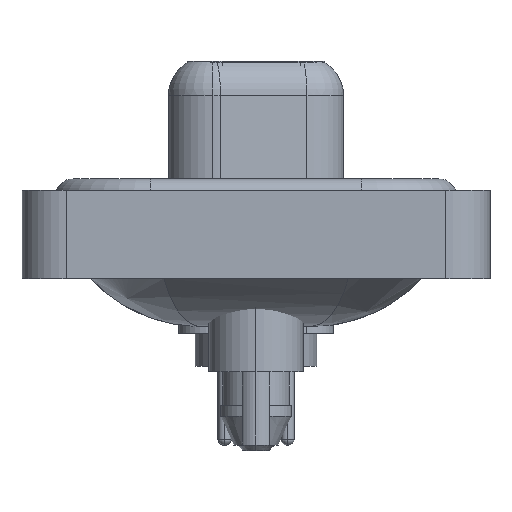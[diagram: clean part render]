
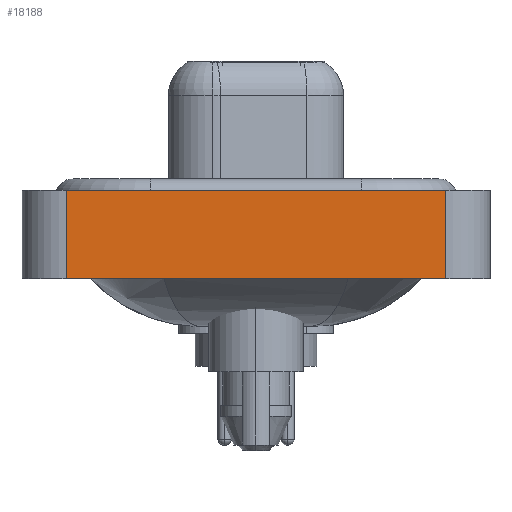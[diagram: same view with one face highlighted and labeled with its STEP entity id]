
A CAD part, left-side view. The second image highlights one B-rep face of the part: STEP entity #18188.
In plain terms, the highlighted planar face has unit normal (-1, 0, 0).
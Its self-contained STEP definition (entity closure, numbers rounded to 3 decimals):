
#572 = LINE ( 'NONE', #20078, #4988 ) ;
#747 = CARTESIAN_POINT ( 'NONE',  ( -7.3, -8.55, -3.6 ) ) ;
#1135 = DIRECTION ( 'NONE',  ( -1., 0., 0. ) ) ;
#1387 = ORIENTED_EDGE ( 'NONE', *, *, #3869, .F. ) ;
#1895 = ORIENTED_EDGE ( 'NONE', *, *, #16898, .T. ) ;
#2384 = CARTESIAN_POINT ( 'NONE',  ( -7.3, -8.55, -3.6 ) ) ;
#3869 = EDGE_CURVE ( 'NONE', #11544, #11591, #7584, .T. ) ;
#3979 = DIRECTION ( 'NONE',  ( 0., -1., 0. ) ) ;
#4447 = DIRECTION ( 'NONE',  ( 0., 0., 1. ) ) ;
#4988 = VECTOR ( 'NONE', #10005, 1000. ) ;
#5085 = DIRECTION ( 'NONE',  ( 0., 0., 1. ) ) ;
#5237 = EDGE_CURVE ( 'NONE', #11591, #5528, #572, .T. ) ;
#5300 = CARTESIAN_POINT ( 'NONE',  ( -7.3, -8.55, -3.6 ) ) ;
#5528 = VERTEX_POINT ( 'NONE', #17703 ) ;
#5994 = VECTOR ( 'NONE', #3979, 1000. ) ;
#6463 = EDGE_CURVE ( 'NONE', #11544, #11216, #18640, .T. ) ;
#7112 = ORIENTED_EDGE ( 'NONE', *, *, #6463, .T. ) ;
#7418 = VECTOR ( 'NONE', #5085, 1000. ) ;
#7584 = LINE ( 'NONE', #10889, #20304 ) ;
#7925 = ORIENTED_EDGE ( 'NONE', *, *, #5237, .F. ) ;
#8734 = LINE ( 'NONE', #5300, #7418 ) ;
#8889 = CARTESIAN_POINT ( 'NONE',  ( -7.3, 8.55, 0.4 ) ) ;
#10005 = DIRECTION ( 'NONE',  ( 0., -1., 0. ) ) ;
#10889 = CARTESIAN_POINT ( 'NONE',  ( -7.3, 8.55, -3.6 ) ) ;
#11216 = VERTEX_POINT ( 'NONE', #2384 ) ;
#11544 = VERTEX_POINT ( 'NONE', #13918 ) ;
#11591 = VERTEX_POINT ( 'NONE', #8889 ) ;
#13786 = FACE_OUTER_BOUND ( 'NONE', #17816, .T. ) ;
#13918 = CARTESIAN_POINT ( 'NONE',  ( -7.3, 8.55, -3.6 ) ) ;
#14002 = DIRECTION ( 'NONE',  ( 0., 0., 1. ) ) ;
#16898 = EDGE_CURVE ( 'NONE', #11216, #5528, #8734, .T. ) ;
#17206 = PLANE ( 'NONE',  #20814 ) ;
#17308 = CARTESIAN_POINT ( 'NONE',  ( -7.3, -8.55, -3.6 ) ) ;
#17703 = CARTESIAN_POINT ( 'NONE',  ( -7.3, -8.55, 0.4 ) ) ;
#17816 = EDGE_LOOP ( 'NONE', ( #1895, #7925, #1387, #7112 ) ) ;
#18188 = ADVANCED_FACE ( 'NONE', ( #13786 ), #17206, .T. ) ;
#18640 = LINE ( 'NONE', #747, #5994 ) ;
#20078 = CARTESIAN_POINT ( 'NONE',  ( -7.3, -8.55, 0.4 ) ) ;
#20304 = VECTOR ( 'NONE', #14002, 1000. ) ;
#20814 = AXIS2_PLACEMENT_3D ( 'NONE', #17308, #1135, #4447 ) ;
